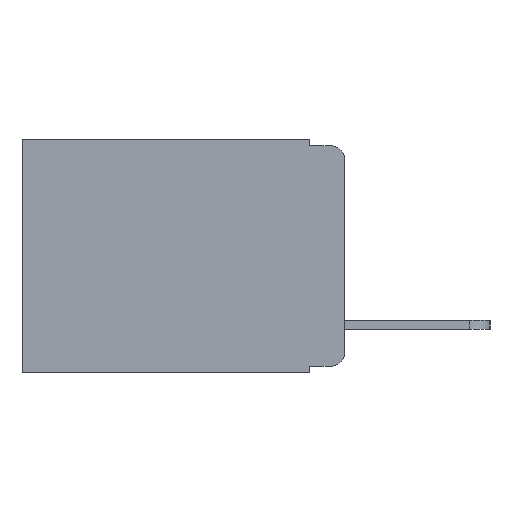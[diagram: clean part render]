
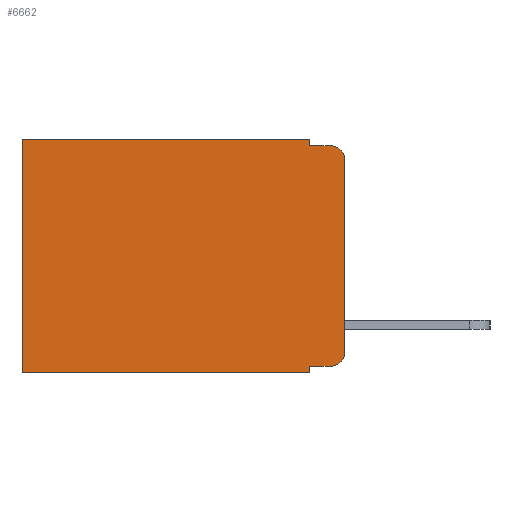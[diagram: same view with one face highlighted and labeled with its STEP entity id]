
A CAD part, left-side view. The second image highlights one B-rep face of the part: STEP entity #6662.
In plain terms, the highlighted planar face has unit normal (-1, 0, 0).
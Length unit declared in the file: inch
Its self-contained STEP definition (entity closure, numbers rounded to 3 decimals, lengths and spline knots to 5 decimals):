
#5 = ORIENTED_EDGE ( 'NONE', *, *, #5669, .F. ) ;
#357 = LINE ( 'NONE', #9299, #11133 ) ;
#387 = VERTEX_POINT ( 'NONE', #5805 ) ;
#417 = ORIENTED_EDGE ( 'NONE', *, *, #5734, .T. ) ;
#532 = DIRECTION ( 'NONE',  ( 0., 0., -1. ) ) ;
#546 = CARTESIAN_POINT ( 'NONE',  ( 0.298, 0.02, -0.333 ) ) ;
#550 = DIRECTION ( 'NONE',  ( 0., 0., -1. ) ) ;
#760 = CARTESIAN_POINT ( 'NONE',  ( 0.298, 0., -0.03 ) ) ;
#961 = VERTEX_POINT ( 'NONE', #11347 ) ;
#1008 = VERTEX_POINT ( 'NONE', #6272 ) ;
#1163 = VERTEX_POINT ( 'NONE', #3527 ) ;
#1425 = EDGE_CURVE ( 'NONE', #10491, #1163, #2651, .T. ) ;
#1474 = DIRECTION ( 'NONE',  ( 0., 0., -1. ) ) ;
#1543 = CARTESIAN_POINT ( 'NONE',  ( 0.298, 0.02, -0.03 ) ) ;
#1549 = DIRECTION ( 'NONE',  ( -1., 0., 0. ) ) ;
#1913 = VERTEX_POINT ( 'NONE', #4050 ) ;
#2426 = CARTESIAN_POINT ( 'NONE',  ( 0.298, 0., 0. ) ) ;
#2500 = LINE ( 'NONE', #3587, #12669 ) ;
#2643 = VECTOR ( 'NONE', #9440, 39.37008 ) ;
#2651 = LINE ( 'NONE', #2426, #12769 ) ;
#3295 = ORIENTED_EDGE ( 'NONE', *, *, #9425, .T. ) ;
#3527 = CARTESIAN_POINT ( 'NONE',  ( 0.298, 0., -0.313 ) ) ;
#3587 = CARTESIAN_POINT ( 'NONE',  ( 0.298, 0.051, -0.333 ) ) ;
#3723 = PLANE ( 'NONE',  #10818 ) ;
#3832 = CARTESIAN_POINT ( 'NONE',  ( 0.298, 0., -0.343 ) ) ;
#4050 = CARTESIAN_POINT ( 'NONE',  ( 0.298, 0.051, -0.343 ) ) ;
#4203 = CARTESIAN_POINT ( 'NONE',  ( 0.298, 0., 0. ) ) ;
#4549 = DIRECTION ( 'NONE',  ( 0., 0., -1. ) ) ;
#4683 = ORIENTED_EDGE ( 'NONE', *, *, #9176, .T. ) ;
#4897 = ORIENTED_EDGE ( 'NONE', *, *, #12113, .T. ) ;
#5488 = LINE ( 'NONE', #3832, #2643 ) ;
#5506 = ORIENTED_EDGE ( 'NONE', *, *, #5654, .T. ) ;
#5654 = EDGE_CURVE ( 'NONE', #1008, #387, #6455, .T. ) ;
#5662 = VECTOR ( 'NONE', #7509, 39.37008 ) ;
#5669 = EDGE_CURVE ( 'NONE', #9575, #1913, #357, .T. ) ;
#5734 = EDGE_CURVE ( 'NONE', #10491, #10560, #8152, .T. ) ;
#5805 = CARTESIAN_POINT ( 'NONE',  ( 0.298, 0.473, -0.343 ) ) ;
#6010 = ORIENTED_EDGE ( 'NONE', *, *, #9119, .F. ) ;
#6151 = CARTESIAN_POINT ( 'NONE',  ( 0.298, 0.051, -0.333 ) ) ;
#6210 = VECTOR ( 'NONE', #11852, 39.37008 ) ;
#6272 = CARTESIAN_POINT ( 'NONE',  ( 0.298, 0.473, 0. ) ) ;
#6455 = LINE ( 'NONE', #8291, #11433 ) ;
#6662 = ADVANCED_FACE ( 'NONE', ( #12472 ), #3723, .F. ) ;
#6871 = AXIS2_PLACEMENT_3D ( 'NONE', #1543, #1549, #1474 ) ;
#6976 = ORIENTED_EDGE ( 'NONE', *, *, #1425, .F. ) ;
#7213 = VECTOR ( 'NONE', #12970, 39.37008 ) ;
#7322 = EDGE_CURVE ( 'NONE', #8646, #961, #9871, .T. ) ;
#7509 = DIRECTION ( 'NONE',  ( 0., -1., 0. ) ) ;
#8152 = CIRCLE ( 'NONE', #6871, 0.02 ) ;
#8236 = LINE ( 'NONE', #12254, #5662 ) ;
#8247 = CARTESIAN_POINT ( 'NONE',  ( 0.298, 0.051, 0. ) ) ;
#8271 = CARTESIAN_POINT ( 'NONE',  ( 0.298, 0.02, -0.313 ) ) ;
#8291 = CARTESIAN_POINT ( 'NONE',  ( 0.298, 0.473, 0. ) ) ;
#8443 = DIRECTION ( 'NONE',  ( -1., 0., 0. ) ) ;
#8646 = VERTEX_POINT ( 'NONE', #8247 ) ;
#9119 = EDGE_CURVE ( 'NONE', #961, #10560, #8236, .T. ) ;
#9176 = EDGE_CURVE ( 'NONE', #9575, #11970, #2500, .T. ) ;
#9211 = CARTESIAN_POINT ( 'NONE',  ( 0.298, 0.051, 0. ) ) ;
#9272 = DIRECTION ( 'NONE',  ( 0., 0., -1. ) ) ;
#9299 = CARTESIAN_POINT ( 'NONE',  ( 0.298, 0.051, 0. ) ) ;
#9425 = EDGE_CURVE ( 'NONE', #11970, #1163, #12551, .T. ) ;
#9440 = DIRECTION ( 'NONE',  ( 0., 1., 0. ) ) ;
#9575 = VERTEX_POINT ( 'NONE', #6151 ) ;
#9686 = ORIENTED_EDGE ( 'NONE', *, *, #7322, .F. ) ;
#9871 = LINE ( 'NONE', #9211, #7213 ) ;
#10337 = ORIENTED_EDGE ( 'NONE', *, *, #11950, .F. ) ;
#10425 = AXIS2_PLACEMENT_3D ( 'NONE', #8271, #8443, #4549 ) ;
#10439 = EDGE_LOOP ( 'NONE', ( #6976, #417, #6010, #9686, #4897, #5506, #10337, #5, #4683, #3295 ) ) ;
#10491 = VERTEX_POINT ( 'NONE', #760 ) ;
#10560 = VERTEX_POINT ( 'NONE', #12298 ) ;
#10818 = AXIS2_PLACEMENT_3D ( 'NONE', #11127, #12438, #11362 ) ;
#11127 = CARTESIAN_POINT ( 'NONE',  ( 0.298, 0., 0. ) ) ;
#11133 = VECTOR ( 'NONE', #532, 39.37008 ) ;
#11347 = CARTESIAN_POINT ( 'NONE',  ( 0.298, 0.051, -0.01 ) ) ;
#11362 = DIRECTION ( 'NONE',  ( 0., 0., -1. ) ) ;
#11433 = VECTOR ( 'NONE', #9272, 39.37008 ) ;
#11481 = LINE ( 'NONE', #4203, #6210 ) ;
#11852 = DIRECTION ( 'NONE',  ( 0., 1., 0. ) ) ;
#11950 = EDGE_CURVE ( 'NONE', #1913, #387, #5488, .T. ) ;
#11970 = VERTEX_POINT ( 'NONE', #546 ) ;
#12044 = DIRECTION ( 'NONE',  ( 0., -1., 0. ) ) ;
#12113 = EDGE_CURVE ( 'NONE', #8646, #1008, #11481, .T. ) ;
#12254 = CARTESIAN_POINT ( 'NONE',  ( 0.298, 0.051, -0.01 ) ) ;
#12298 = CARTESIAN_POINT ( 'NONE',  ( 0.298, 0.02, -0.01 ) ) ;
#12438 = DIRECTION ( 'NONE',  ( 1., 0., 0. ) ) ;
#12472 = FACE_OUTER_BOUND ( 'NONE', #10439, .T. ) ;
#12551 = CIRCLE ( 'NONE', #10425, 0.02 ) ;
#12669 = VECTOR ( 'NONE', #12044, 39.37008 ) ;
#12769 = VECTOR ( 'NONE', #550, 39.37008 ) ;
#12970 = DIRECTION ( 'NONE',  ( 0., 0., -1. ) ) ;
